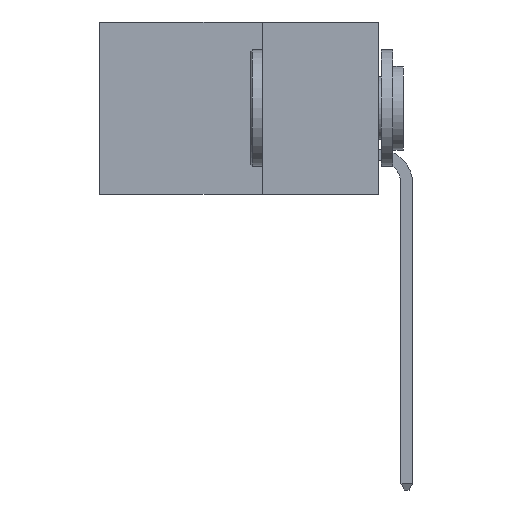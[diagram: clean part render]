
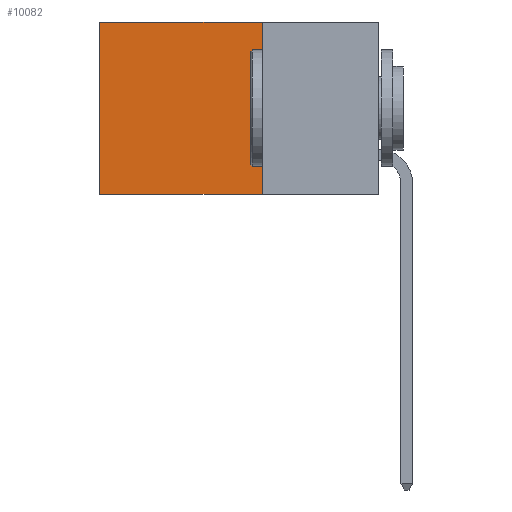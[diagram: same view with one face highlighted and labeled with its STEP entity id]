
A CAD part, left-side view. The second image highlights one B-rep face of the part: STEP entity #10082.
In plain terms, the highlighted planar face has unit normal (-1, 0, 0).
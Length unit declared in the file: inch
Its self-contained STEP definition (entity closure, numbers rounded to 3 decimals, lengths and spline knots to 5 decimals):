
#1214 = LINE ( 'NONE', #6462, #14869 ) ;
#1706 = CARTESIAN_POINT ( 'NONE',  ( 0.2615, 0.6, -0.37 ) ) ;
#1821 = EDGE_CURVE ( 'NONE', #19340, #15270, #1214, .T. ) ;
#2501 = LINE ( 'NONE', #19502, #11471 ) ;
#4127 = LINE ( 'NONE', #4992, #8368 ) ;
#4992 = CARTESIAN_POINT ( 'NONE',  ( 0.2615, 0.6, -0.37 ) ) ;
#5130 = LINE ( 'NONE', #9812, #8765 ) ;
#6008 = ORIENTED_EDGE ( 'NONE', *, *, #12460, .F. ) ;
#6462 = CARTESIAN_POINT ( 'NONE',  ( 0.2615, 0.25, 0. ) ) ;
#6547 = DIRECTION ( 'NONE',  ( 0., 1., 0. ) ) ;
#8368 = VECTOR ( 'NONE', #8669, 39.37008 ) ;
#8669 = DIRECTION ( 'NONE',  ( 0., 0., -1. ) ) ;
#8765 = VECTOR ( 'NONE', #9766, 39.37008 ) ;
#9766 = DIRECTION ( 'NONE',  ( 0., 0., -1. ) ) ;
#9812 = CARTESIAN_POINT ( 'NONE',  ( 0.2615, 0.25, -0.37 ) ) ;
#10082 = ADVANCED_FACE ( 'NONE', ( #11389 ), #12741, .F. ) ;
#11389 = FACE_OUTER_BOUND ( 'NONE', #16084, .T. ) ;
#11471 = VECTOR ( 'NONE', #21133, 39.37008 ) ;
#12460 = EDGE_CURVE ( 'NONE', #19340, #17419, #5130, .T. ) ;
#12464 = DIRECTION ( 'NONE',  ( 0., 0., -1. ) ) ;
#12536 = AXIS2_PLACEMENT_3D ( 'NONE', #12665, #12620, #12464 ) ;
#12620 = DIRECTION ( 'NONE',  ( 1., 0., 0. ) ) ;
#12665 = CARTESIAN_POINT ( 'NONE',  ( 0.2615, 0.25, -0.37 ) ) ;
#12741 = PLANE ( 'NONE',  #12536 ) ;
#13855 = CARTESIAN_POINT ( 'NONE',  ( 0.2615, 0.6, 0. ) ) ;
#14869 = VECTOR ( 'NONE', #6547, 39.37008 ) ;
#15153 = CARTESIAN_POINT ( 'NONE',  ( 0.2615, 0.25, 0. ) ) ;
#15270 = VERTEX_POINT ( 'NONE', #13855 ) ;
#15272 = ORIENTED_EDGE ( 'NONE', *, *, #19518, .T. ) ;
#16084 = EDGE_LOOP ( 'NONE', ( #15272, #20216, #6008, #20720 ) ) ;
#16660 = CARTESIAN_POINT ( 'NONE',  ( 0.2615, 0.25, -0.37 ) ) ;
#17419 = VERTEX_POINT ( 'NONE', #16660 ) ;
#19340 = VERTEX_POINT ( 'NONE', #15153 ) ;
#19502 = CARTESIAN_POINT ( 'NONE',  ( 0.2615, 0.25, -0.37 ) ) ;
#19518 = EDGE_CURVE ( 'NONE', #15270, #20300, #4127, .T. ) ;
#20216 = ORIENTED_EDGE ( 'NONE', *, *, #22565, .F. ) ;
#20300 = VERTEX_POINT ( 'NONE', #1706 ) ;
#20720 = ORIENTED_EDGE ( 'NONE', *, *, #1821, .T. ) ;
#21133 = DIRECTION ( 'NONE',  ( 0., 1., 0. ) ) ;
#22565 = EDGE_CURVE ( 'NONE', #17419, #20300, #2501, .T. ) ;
